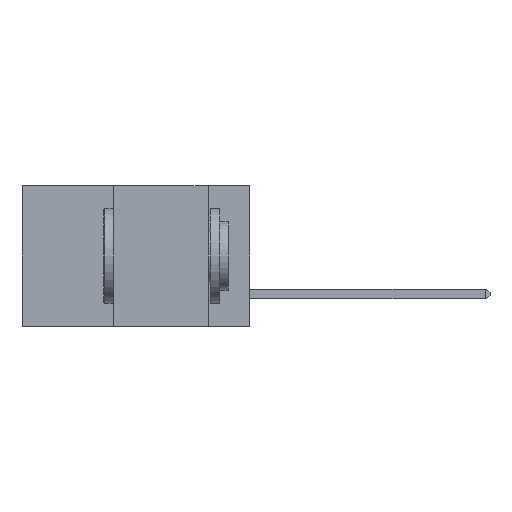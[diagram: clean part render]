
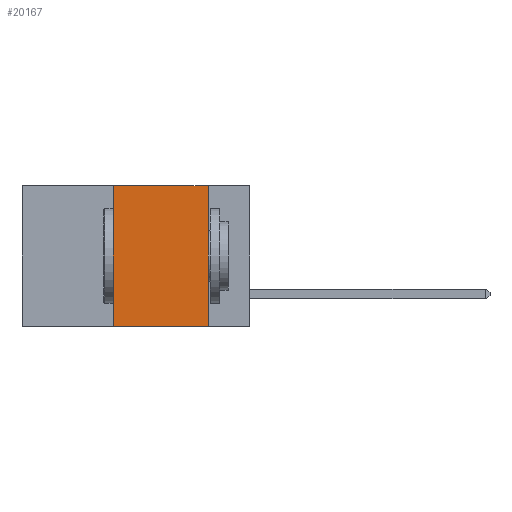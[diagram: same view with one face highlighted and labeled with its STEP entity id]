
A CAD part, left-side view. The second image highlights one B-rep face of the part: STEP entity #20167.
In plain terms, the highlighted planar face has unit normal (-1, 0, 0).
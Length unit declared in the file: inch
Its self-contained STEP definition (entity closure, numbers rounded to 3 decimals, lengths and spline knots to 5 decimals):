
#494 = VECTOR ( 'NONE', #2026, 39.37008 ) ;
#907 = LINE ( 'NONE', #21536, #17811 ) ;
#1484 = DIRECTION ( 'NONE',  ( 0., 0., -1. ) ) ;
#1528 = LINE ( 'NONE', #17851, #494 ) ;
#2026 = DIRECTION ( 'NONE',  ( 0., -1., 0. ) ) ;
#2592 = DIRECTION ( 'NONE',  ( 0., 0., 1. ) ) ;
#3186 = FACE_OUTER_BOUND ( 'NONE', #23767, .T. ) ;
#4289 = VERTEX_POINT ( 'NONE', #4955 ) ;
#4788 = VERTEX_POINT ( 'NONE', #29090 ) ;
#4955 = CARTESIAN_POINT ( 'NONE',  ( 0., 0.36, 0. ) ) ;
#5428 = CARTESIAN_POINT ( 'NONE',  ( 0., 0.11, 0. ) ) ;
#7041 = ORIENTED_EDGE ( 'NONE', *, *, #7263, .T. ) ;
#7263 = EDGE_CURVE ( 'NONE', #4788, #37025, #1528, .T. ) ;
#8349 = DIRECTION ( 'NONE',  ( 0., -1., 0. ) ) ;
#13578 = EDGE_CURVE ( 'NONE', #39293, #37025, #39294, .T. ) ;
#14495 = ORIENTED_EDGE ( 'NONE', *, *, #37432, .F. ) ;
#15829 = CARTESIAN_POINT ( 'NONE',  ( 0., 0.11, -0.37 ) ) ;
#17811 = VECTOR ( 'NONE', #2592, 39.37008 ) ;
#17851 = CARTESIAN_POINT ( 'NONE',  ( 0., 0.6, -0.37 ) ) ;
#18290 = LINE ( 'NONE', #23911, #25519 ) ;
#20167 = ADVANCED_FACE ( 'NONE', ( #3186 ), #35760, .F. ) ;
#20424 = DIRECTION ( 'NONE',  ( 1., 0., 0. ) ) ;
#21536 = CARTESIAN_POINT ( 'NONE',  ( 0., 0.36, 0. ) ) ;
#22801 = EDGE_CURVE ( 'NONE', #4289, #39293, #18290, .T. ) ;
#22955 = VECTOR ( 'NONE', #24217, 39.37008 ) ;
#23767 = EDGE_LOOP ( 'NONE', ( #27038, #29933, #14495, #7041 ) ) ;
#23911 = CARTESIAN_POINT ( 'NONE',  ( 0., 0.6, 0. ) ) ;
#24217 = DIRECTION ( 'NONE',  ( 0., 0., -1. ) ) ;
#25519 = VECTOR ( 'NONE', #8349, 39.37008 ) ;
#27038 = ORIENTED_EDGE ( 'NONE', *, *, #13578, .F. ) ;
#29090 = CARTESIAN_POINT ( 'NONE',  ( 0., 0.36, -0.37 ) ) ;
#29933 = ORIENTED_EDGE ( 'NONE', *, *, #22801, .F. ) ;
#30830 = AXIS2_PLACEMENT_3D ( 'NONE', #38844, #20424, #1484 ) ;
#35760 = PLANE ( 'NONE',  #30830 ) ;
#37025 = VERTEX_POINT ( 'NONE', #15829 ) ;
#37432 = EDGE_CURVE ( 'NONE', #4788, #4289, #907, .T. ) ;
#38844 = CARTESIAN_POINT ( 'NONE',  ( 0., 0.6, 0. ) ) ;
#39293 = VERTEX_POINT ( 'NONE', #39646 ) ;
#39294 = LINE ( 'NONE', #5428, #22955 ) ;
#39646 = CARTESIAN_POINT ( 'NONE',  ( 0., 0.11, 0. ) ) ;
